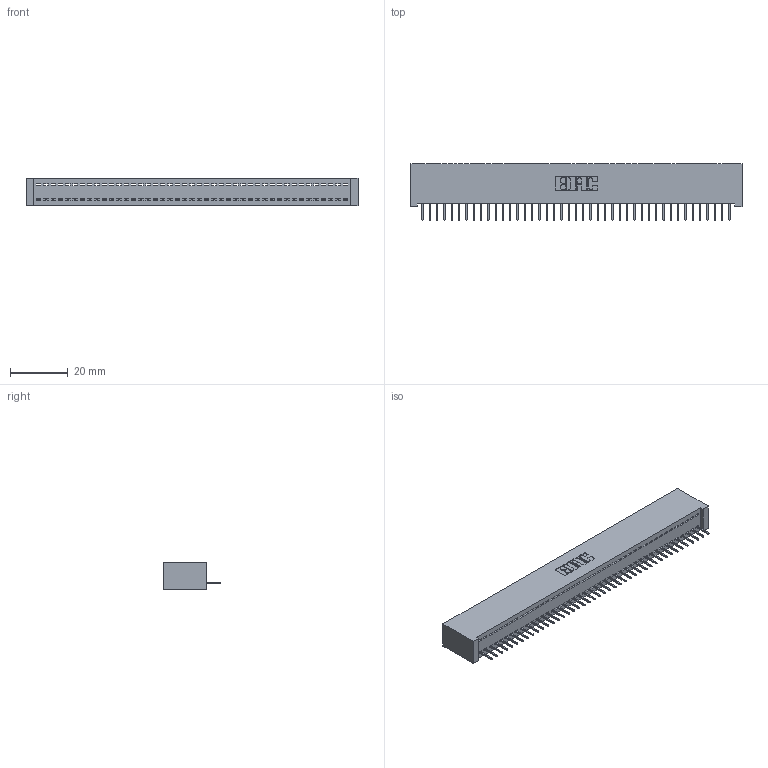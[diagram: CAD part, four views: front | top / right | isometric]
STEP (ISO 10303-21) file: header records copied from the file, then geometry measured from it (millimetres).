
FILE_DESCRIPTION (( 'STEP AP203' ), '1' );
FILE_NAME ('342-043-524-101.STEP', '2018-08-12T13:47:08', ( '' ), ( '' ), 'SwSTEP 2.0', 'SolidWorks 2016', '' );
FILE_SCHEMA (( 'CONFIG_CONTROL_DESIGN' ));
Length unit declared in the file: inch
Products named in the file (3): 342 Part_Lugless; 345-292-001_345-293-124; 342-043-524-101
Assembly tree (44 placements, depth 2):
  342-043-524-101
    342 Part_Lugless
    345-292-001_345-293-124  x43
Bounding box: 115.47 x 19.69 x 9.4 mm (x, y, z)
Volume: 10367.1 mm3; surface area: 15037.9 mm2
Topology: 44 solids, 44 shells, 2768 faces, 8015 edges, 5170 vertices
Faces by surface type: plane 2126, cylinder 642
Entity records: 25823 total; most frequent: CARTESIAN_POINT 4459, ORIENTED_EDGE 4438, DIRECTION 3753, EDGE_CURVE 2219, VECTOR 2103, LINE 2103, VERTEX_POINT 1474, AXIS2_PLACEMENT_3D 825
